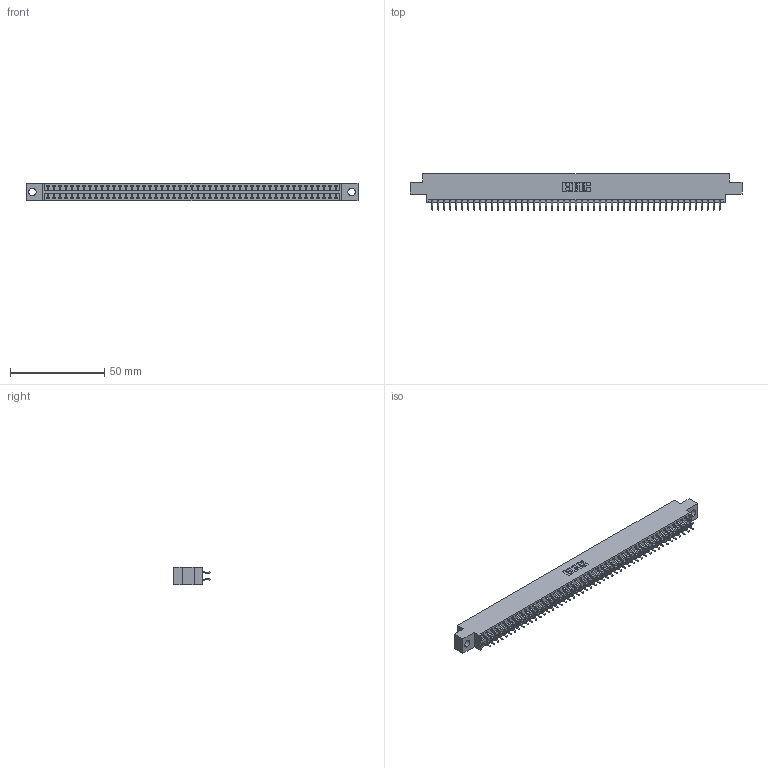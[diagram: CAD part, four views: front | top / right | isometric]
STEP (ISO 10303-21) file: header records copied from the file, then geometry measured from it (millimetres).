
FILE_DESCRIPTION (( 'STEP AP203' ), '1' );
FILE_NAME ('346-098-556-804.STEP', '2022-05-26T18:58:02', ( '' ), ( '' ), 'SwSTEP 2.0', 'SolidWorks 2020', '' );
FILE_SCHEMA (( 'CONFIG_CONTROL_DESIGN' ));
Length unit declared in the file: inch
Products named in the file (3): 345-292-001_556 Tail; 346 Part_0.170 Offset - 0.156 Dia-TH; 346-098-556-804
Assembly tree (99 placements, depth 2):
  346-098-556-804
    346 Part_0.170 Offset - 0.156 Dia-TH
    345-292-001_556 Tail  x98
Bounding box: 176.15 x 19.57 x 9.4 mm (x, y, z)
Volume: 16966.6 mm3; surface area: 23368.3 mm2
Topology: 99 solids, 99 shells, 5824 faces, 17331 edges, 11422 vertices
Faces by surface type: plane 3916, cylinder 1908
Entity records: 31807 total; most frequent: CARTESIAN_POINT 5254, ORIENTED_EDGE 5174, DIRECTION 4667, EDGE_CURVE 2587, LINE 2251, VECTOR 2251, VERTEX_POINT 1722, AXIS2_PLACEMENT_3D 1208
